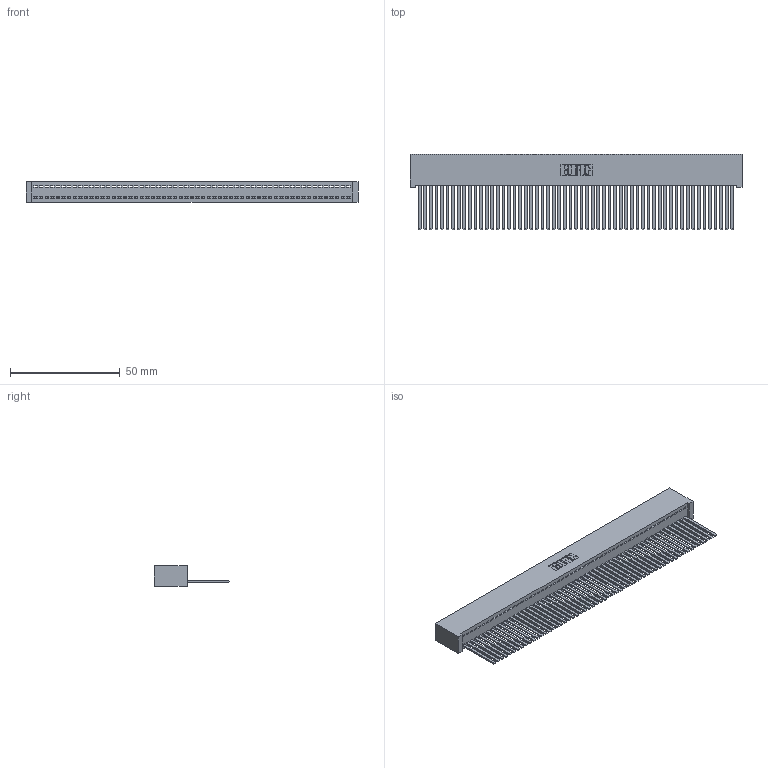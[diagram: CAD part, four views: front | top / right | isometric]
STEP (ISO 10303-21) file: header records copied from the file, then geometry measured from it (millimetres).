
FILE_DESCRIPTION (( 'STEP AP203' ), '1' );
FILE_NAME ('342-057-544-101.STEP', '2018-08-13T04:37:35', ( '' ), ( '' ), 'SwSTEP 2.0', 'SolidWorks 2016', '' );
FILE_SCHEMA (( 'CONFIG_CONTROL_DESIGN' ));
Length unit declared in the file: inch
Products named in the file (3): 342 Part_Lugless; 345-292-001_345-293-144; 342-057-544-101
Assembly tree (58 placements, depth 2):
  342-057-544-101
    342 Part_Lugless
    345-292-001_345-293-144  x57
Bounding box: 151.03 x 34.3 x 9.4 mm (x, y, z)
Volume: 14366.5 mm3; surface area: 23578.8 mm2
Topology: 58 solids, 58 shells, 3066 faces, 9281 edges, 6110 vertices
Faces by surface type: plane 2228, cylinder 838
Entity records: 32313 total; most frequent: CARTESIAN_POINT 5577, ORIENTED_EDGE 5570, DIRECTION 4663, EDGE_CURVE 2785, VECTOR 2669, LINE 2669, VERTEX_POINT 1854, AXIS2_PLACEMENT_3D 997
